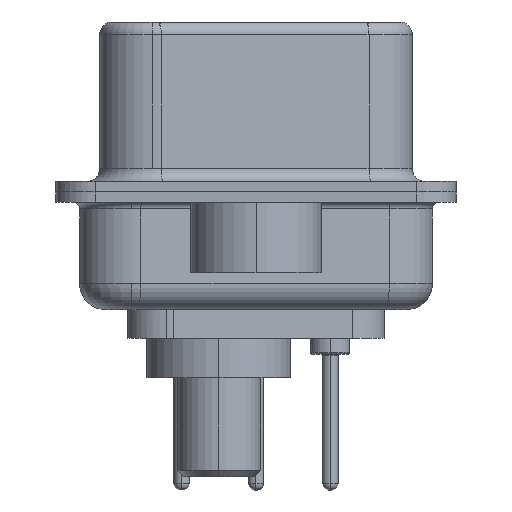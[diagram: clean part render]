
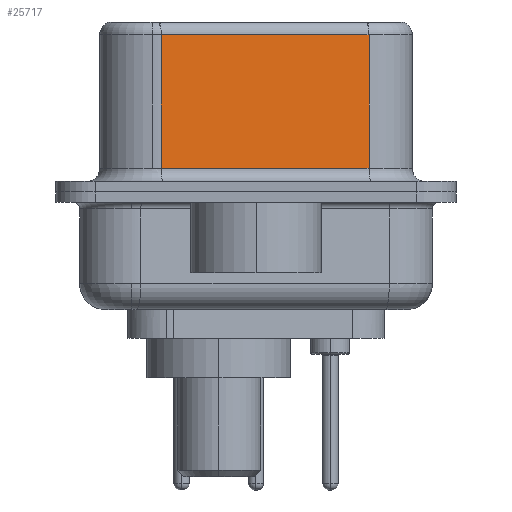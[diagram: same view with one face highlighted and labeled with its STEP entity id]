
A CAD part, left-side view. The second image highlights one B-rep face of the part: STEP entity #25717.
In plain terms, the highlighted planar face has unit normal (-0.985, -0.174, 0).
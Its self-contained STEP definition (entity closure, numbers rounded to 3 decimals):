
#1183 = VERTEX_POINT ( 'NONE', #15866 ) ;
#1302 = EDGE_LOOP ( 'NONE', ( #20779, #18500, #1908, #20807 ) ) ;
#1908 = ORIENTED_EDGE ( 'NONE', *, *, #8387, .T. ) ;
#2001 = VERTEX_POINT ( 'NONE', #13716 ) ;
#4503 = LINE ( 'NONE', #26398, #25577 ) ;
#5576 = CARTESIAN_POINT ( 'NONE',  ( 5.132, -4.322, 6.52 ) ) ;
#6005 = DIRECTION ( 'NONE',  ( 0.174, -0.985, 0. ) ) ;
#6713 = CARTESIAN_POINT ( 'NONE',  ( 3.73, 3.628, 6.52 ) ) ;
#6745 = DIRECTION ( 'NONE',  ( 0., 0., -1. ) ) ;
#6888 = VECTOR ( 'NONE', #17746, 1000. ) ;
#6977 = CARTESIAN_POINT ( 'NONE',  ( 5.132, -4.322, 6.02 ) ) ;
#8051 = CARTESIAN_POINT ( 'NONE',  ( 5.132, -4.322, 0.9 ) ) ;
#8387 = EDGE_CURVE ( 'NONE', #1183, #2001, #23800, .T. ) ;
#8950 = CARTESIAN_POINT ( 'NONE',  ( 5.132, -4.322, 6.52 ) ) ;
#9097 = LINE ( 'NONE', #5576, #6888 ) ;
#9159 = VECTOR ( 'NONE', #6005, 1000. ) ;
#9820 = AXIS2_PLACEMENT_3D ( 'NONE', #8950, #23284, #10965 ) ;
#10128 = CARTESIAN_POINT ( 'NONE',  ( 5.132, -4.322, 0.9 ) ) ;
#10965 = DIRECTION ( 'NONE',  ( -0.174, 0.985, 0. ) ) ;
#12084 = DIRECTION ( 'NONE',  ( -0.174, 0.985, 0. ) ) ;
#12109 = VERTEX_POINT ( 'NONE', #10128 ) ;
#13508 = VECTOR ( 'NONE', #6745, 1000. ) ;
#13716 = CARTESIAN_POINT ( 'NONE',  ( 3.73, 3.628, 0.9 ) ) ;
#15866 = CARTESIAN_POINT ( 'NONE',  ( 3.73, 3.628, 6.02 ) ) ;
#16473 = EDGE_CURVE ( 'NONE', #21483, #12109, #9097, .T. ) ;
#17746 = DIRECTION ( 'NONE',  ( 0., 0., -1. ) ) ;
#18155 = FACE_OUTER_BOUND ( 'NONE', #1302, .T. ) ;
#18500 = ORIENTED_EDGE ( 'NONE', *, *, #19038, .T. ) ;
#19038 = EDGE_CURVE ( 'NONE', #21483, #1183, #4503, .T. ) ;
#20779 = ORIENTED_EDGE ( 'NONE', *, *, #16473, .F. ) ;
#20807 = ORIENTED_EDGE ( 'NONE', *, *, #21179, .T. ) ;
#21179 = EDGE_CURVE ( 'NONE', #2001, #12109, #24842, .T. ) ;
#21211 = PLANE ( 'NONE',  #9820 ) ;
#21483 = VERTEX_POINT ( 'NONE', #6977 ) ;
#23284 = DIRECTION ( 'NONE',  ( 0.985, 0.174, 0. ) ) ;
#23800 = LINE ( 'NONE', #6713, #13508 ) ;
#24842 = LINE ( 'NONE', #8051, #9159 ) ;
#25577 = VECTOR ( 'NONE', #12084, 1000. ) ;
#25717 = ADVANCED_FACE ( 'NONE', ( #18155 ), #21211, .F. ) ;
#26398 = CARTESIAN_POINT ( 'NONE',  ( 5.132, -4.322, 6.02 ) ) ;
